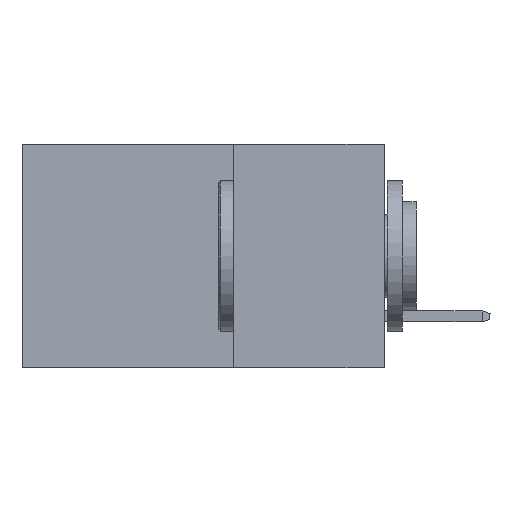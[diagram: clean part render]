
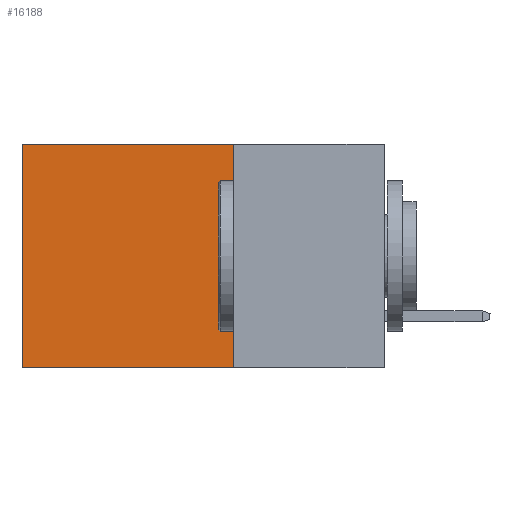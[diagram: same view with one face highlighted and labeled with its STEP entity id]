
A CAD part, left-side view. The second image highlights one B-rep face of the part: STEP entity #16188.
In plain terms, the highlighted planar face has unit normal (-1, 0, 0).
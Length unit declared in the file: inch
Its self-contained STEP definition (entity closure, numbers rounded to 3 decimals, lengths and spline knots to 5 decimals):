
#41 = LINE ( 'NONE', #7355, #23212 ) ;
#466 = DIRECTION ( 'NONE',  ( 0., 0., -1. ) ) ;
#884 = ORIENTED_EDGE ( 'NONE', *, *, #8636, .F. ) ;
#1512 = EDGE_CURVE ( 'NONE', #18118, #20584, #17079, .T. ) ;
#2526 = ORIENTED_EDGE ( 'NONE', *, *, #24131, .T. ) ;
#2769 = EDGE_LOOP ( 'NONE', ( #2526, #884, #15834, #9501 ) ) ;
#2866 = VERTEX_POINT ( 'NONE', #19173 ) ;
#3185 = DIRECTION ( 'NONE',  ( 0., 0., -1. ) ) ;
#3677 = CARTESIAN_POINT ( 'NONE',  ( 0.2615, 0.6, 0. ) ) ;
#5877 = LINE ( 'NONE', #7614, #18412 ) ;
#7355 = CARTESIAN_POINT ( 'NONE',  ( 0.2615, 0.25, 0. ) ) ;
#7614 = CARTESIAN_POINT ( 'NONE',  ( 0.2615, 0.25, -0.37 ) ) ;
#7968 = CARTESIAN_POINT ( 'NONE',  ( 0.2615, 0.6, -0.37 ) ) ;
#8562 = AXIS2_PLACEMENT_3D ( 'NONE', #21432, #12044, #3185 ) ;
#8636 = EDGE_CURVE ( 'NONE', #20584, #2866, #5877, .T. ) ;
#9501 = ORIENTED_EDGE ( 'NONE', *, *, #16750, .T. ) ;
#9574 = VECTOR ( 'NONE', #466, 39.37008 ) ;
#9612 = DIRECTION ( 'NONE',  ( 0., 1., 0. ) ) ;
#11349 = DIRECTION ( 'NONE',  ( 0., 1., 0. ) ) ;
#11667 = CARTESIAN_POINT ( 'NONE',  ( 0.2615, 0.25, -0.37 ) ) ;
#12044 = DIRECTION ( 'NONE',  ( 1., 0., 0. ) ) ;
#12067 = LINE ( 'NONE', #7968, #22213 ) ;
#13975 = CARTESIAN_POINT ( 'NONE',  ( 0.2615, 0.25, 0. ) ) ;
#15834 = ORIENTED_EDGE ( 'NONE', *, *, #1512, .F. ) ;
#16188 = ADVANCED_FACE ( 'NONE', ( #19432 ), #22003, .F. ) ;
#16750 = EDGE_CURVE ( 'NONE', #18118, #23488, #41, .T. ) ;
#17079 = LINE ( 'NONE', #11667, #9574 ) ;
#18118 = VERTEX_POINT ( 'NONE', #13975 ) ;
#18412 = VECTOR ( 'NONE', #9612, 39.37008 ) ;
#19173 = CARTESIAN_POINT ( 'NONE',  ( 0.2615, 0.6, -0.37 ) ) ;
#19432 = FACE_OUTER_BOUND ( 'NONE', #2769, .T. ) ;
#20584 = VERTEX_POINT ( 'NONE', #23067 ) ;
#21432 = CARTESIAN_POINT ( 'NONE',  ( 0.2615, 0.25, -0.37 ) ) ;
#22003 = PLANE ( 'NONE',  #8562 ) ;
#22213 = VECTOR ( 'NONE', #23319, 39.37008 ) ;
#23067 = CARTESIAN_POINT ( 'NONE',  ( 0.2615, 0.25, -0.37 ) ) ;
#23212 = VECTOR ( 'NONE', #11349, 39.37008 ) ;
#23319 = DIRECTION ( 'NONE',  ( 0., 0., -1. ) ) ;
#23488 = VERTEX_POINT ( 'NONE', #3677 ) ;
#24131 = EDGE_CURVE ( 'NONE', #23488, #2866, #12067, .T. ) ;
